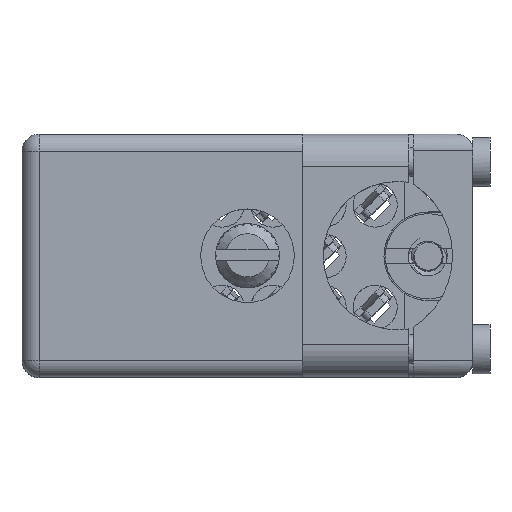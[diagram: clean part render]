
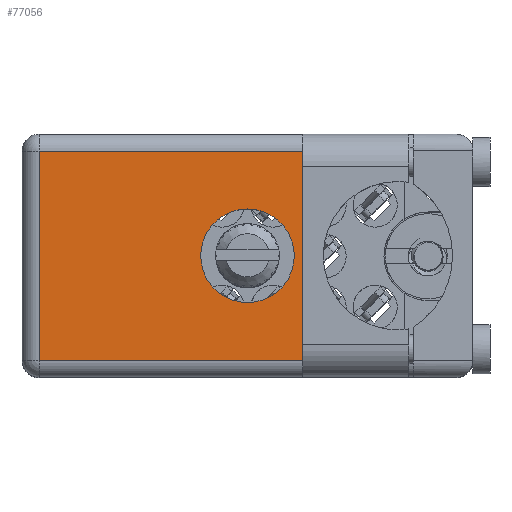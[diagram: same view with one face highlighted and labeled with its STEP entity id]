
A CAD part, top view. The second image highlights one B-rep face of the part: STEP entity #77056.
In plain terms, the highlighted face is planar.
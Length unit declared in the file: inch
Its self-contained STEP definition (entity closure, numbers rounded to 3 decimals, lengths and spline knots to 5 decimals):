
#2816 = FACE_OUTER_BOUND ( 'NONE', #39964, .T. ) ;
#5019 = ORIENTED_EDGE ( 'NONE', *, *, #169925, .T. ) ;
#7229 = VECTOR ( 'NONE', #134610, 39.37008 ) ;
#10296 = DIRECTION ( 'NONE',  ( 1., 0., 0. ) ) ;
#12854 = LINE ( 'NONE', #140086, #100117 ) ;
#14475 = LINE ( 'NONE', #176912, #71023 ) ;
#15348 = ORIENTED_EDGE ( 'NONE', *, *, #32912, .T. ) ;
#18903 = VECTOR ( 'NONE', #10296, 39.37008 ) ;
#21720 = FACE_BOUND ( 'NONE', #161489, .T. ) ;
#24932 = CARTESIAN_POINT ( 'NONE',  ( 1.15, 0.906, -0.05 ) ) ;
#25949 = DIRECTION ( 'NONE',  ( -1., 0., 0. ) ) ;
#26892 = CIRCLE ( 'NONE', #84738, 0.1375 ) ;
#27296 = DIRECTION ( 'NONE',  ( 0., 0., -1. ) ) ;
#27607 = CARTESIAN_POINT ( 'NONE',  ( 0., 0.906, -0.715 ) ) ;
#28486 = LINE ( 'NONE', #96428, #144099 ) ;
#32428 = EDGE_CURVE ( 'NONE', #192081, #61509, #56772, .T. ) ;
#32912 = EDGE_CURVE ( 'NONE', #193799, #192081, #132335, .T. ) ;
#34143 = CIRCLE ( 'NONE', #130358, 0.1375 ) ;
#36052 = VERTEX_POINT ( 'NONE', #110665 ) ;
#37964 = DIRECTION ( 'NONE',  ( 1., 0., 0. ) ) ;
#38659 = ORIENTED_EDGE ( 'NONE', *, *, #109592, .F. ) ;
#39964 = EDGE_LOOP ( 'NONE', ( #15348, #168463, #132855, #195658, #127705, #64110, #38659, #5019 ) ) ;
#43865 = EDGE_CURVE ( 'NONE', #47152, #95052, #26892, .T. ) ;
#47152 = VERTEX_POINT ( 'NONE', #162178 ) ;
#48878 = EDGE_CURVE ( 'NONE', #102136, #36052, #107818, .T. ) ;
#52043 = VECTOR ( 'NONE', #124197, 39.37008 ) ;
#52554 = EDGE_CURVE ( 'NONE', #95052, #47152, #34143, .T. ) ;
#52953 = ORIENTED_EDGE ( 'NONE', *, *, #43865, .F. ) ;
#56772 = LINE ( 'NONE', #145540, #18903 ) ;
#58679 = CARTESIAN_POINT ( 'NONE',  ( 1.15, 0.906, -0.715 ) ) ;
#61509 = VERTEX_POINT ( 'NONE', #24932 ) ;
#64110 = ORIENTED_EDGE ( 'NONE', *, *, #172129, .T. ) ;
#71023 = VECTOR ( 'NONE', #27296, 39.37008 ) ;
#77056 = ADVANCED_FACE ( 'NONE', ( #2816, #21720 ), #88414, .T. ) ;
#83364 = DIRECTION ( 'NONE',  ( 0., 0., 1. ) ) ;
#84738 = AXIS2_PLACEMENT_3D ( 'NONE', #89733, #182481, #194965 ) ;
#86736 = CARTESIAN_POINT ( 'NONE',  ( 0.865, 0.906, -0.1125 ) ) ;
#88414 = PLANE ( 'NONE',  #143368 ) ;
#89733 = CARTESIAN_POINT ( 'NONE',  ( 0.6625, 0.906, -0.3575 ) ) ;
#93908 = CARTESIAN_POINT ( 'NONE',  ( 0.05, 0.906, -0.715 ) ) ;
#95052 = VERTEX_POINT ( 'NONE', #193971 ) ;
#96428 = CARTESIAN_POINT ( 'NONE',  ( 0., 0.906, -0.665 ) ) ;
#98882 = DIRECTION ( 'NONE',  ( 0., 1., 0. ) ) ;
#100117 = VECTOR ( 'NONE', #83364, 39.37008 ) ;
#102136 = VERTEX_POINT ( 'NONE', #160832 ) ;
#107818 = LINE ( 'NONE', #86736, #126714 ) ;
#109592 = EDGE_CURVE ( 'NONE', #149557, #163975, #137191, .T. ) ;
#110665 = CARTESIAN_POINT ( 'NONE',  ( 0.865, 0.906, -0.1125 ) ) ;
#111918 = CARTESIAN_POINT ( 'NONE',  ( 0.865, 0.906, -0.6025 ) ) ;
#124140 = CARTESIAN_POINT ( 'NONE',  ( 1.15, 0.906, -0.6025 ) ) ;
#124197 = DIRECTION ( 'NONE',  ( 0., 0., 1. ) ) ;
#126714 = VECTOR ( 'NONE', #25949, 39.37008 ) ;
#126743 = DIRECTION ( 'NONE',  ( -1., 0., 0. ) ) ;
#127705 = ORIENTED_EDGE ( 'NONE', *, *, #153642, .T. ) ;
#130358 = AXIS2_PLACEMENT_3D ( 'NONE', #183645, #167944, #137043 ) ;
#130460 = ORIENTED_EDGE ( 'NONE', *, *, #52554, .F. ) ;
#132335 = LINE ( 'NONE', #93908, #52043 ) ;
#132855 = ORIENTED_EDGE ( 'NONE', *, *, #180693, .F. ) ;
#133854 = DIRECTION ( 'NONE',  ( 0., 0., 1. ) ) ;
#134610 = DIRECTION ( 'NONE',  ( 0., 0., 1. ) ) ;
#137043 = DIRECTION ( 'NONE',  ( 0., 0., 1. ) ) ;
#137191 = LINE ( 'NONE', #58679, #7229 ) ;
#140086 = CARTESIAN_POINT ( 'NONE',  ( 1.15, 0.906, -0.715 ) ) ;
#143368 = AXIS2_PLACEMENT_3D ( 'NONE', #27607, #98882, #133854 ) ;
#144099 = VECTOR ( 'NONE', #126743, 39.37008 ) ;
#145540 = CARTESIAN_POINT ( 'NONE',  ( 1.15, 0.906, -0.05 ) ) ;
#146742 = VERTEX_POINT ( 'NONE', #147879 ) ;
#147879 = CARTESIAN_POINT ( 'NONE',  ( 0.865, 0.906, -0.6025 ) ) ;
#149557 = VERTEX_POINT ( 'NONE', #188410 ) ;
#153642 = EDGE_CURVE ( 'NONE', #36052, #146742, #14475, .T. ) ;
#160832 = CARTESIAN_POINT ( 'NONE',  ( 1.15, 0.906, -0.1125 ) ) ;
#161489 = EDGE_LOOP ( 'NONE', ( #52953, #130460 ) ) ;
#162178 = CARTESIAN_POINT ( 'NONE',  ( 0.6625, 0.906, -0.22 ) ) ;
#163975 = VERTEX_POINT ( 'NONE', #124140 ) ;
#167944 = DIRECTION ( 'NONE',  ( 0., 1., 0. ) ) ;
#168463 = ORIENTED_EDGE ( 'NONE', *, *, #32428, .T. ) ;
#169925 = EDGE_CURVE ( 'NONE', #149557, #193799, #28486, .T. ) ;
#172129 = EDGE_CURVE ( 'NONE', #146742, #163975, #190719, .T. ) ;
#173573 = CARTESIAN_POINT ( 'NONE',  ( 0.05, 0.906, -0.665 ) ) ;
#176912 = CARTESIAN_POINT ( 'NONE',  ( 0.865, 0.906, -0.1125 ) ) ;
#179014 = VECTOR ( 'NONE', #37964, 39.37008 ) ;
#180693 = EDGE_CURVE ( 'NONE', #102136, #61509, #12854, .T. ) ;
#182481 = DIRECTION ( 'NONE',  ( 0., 1., 0. ) ) ;
#183645 = CARTESIAN_POINT ( 'NONE',  ( 0.6625, 0.906, -0.3575 ) ) ;
#188410 = CARTESIAN_POINT ( 'NONE',  ( 1.15, 0.906, -0.665 ) ) ;
#190719 = LINE ( 'NONE', #111918, #179014 ) ;
#192081 = VERTEX_POINT ( 'NONE', #192712 ) ;
#192712 = CARTESIAN_POINT ( 'NONE',  ( 0.05, 0.906, -0.05 ) ) ;
#193799 = VERTEX_POINT ( 'NONE', #173573 ) ;
#193971 = CARTESIAN_POINT ( 'NONE',  ( 0.6625, 0.906, -0.495 ) ) ;
#194965 = DIRECTION ( 'NONE',  ( 0., 0., 1. ) ) ;
#195658 = ORIENTED_EDGE ( 'NONE', *, *, #48878, .T. ) ;
